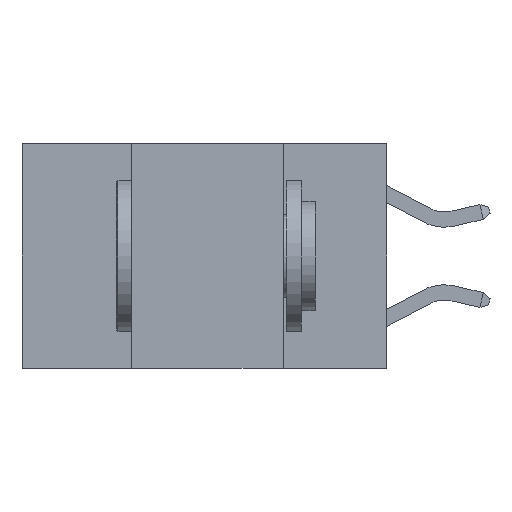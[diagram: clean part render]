
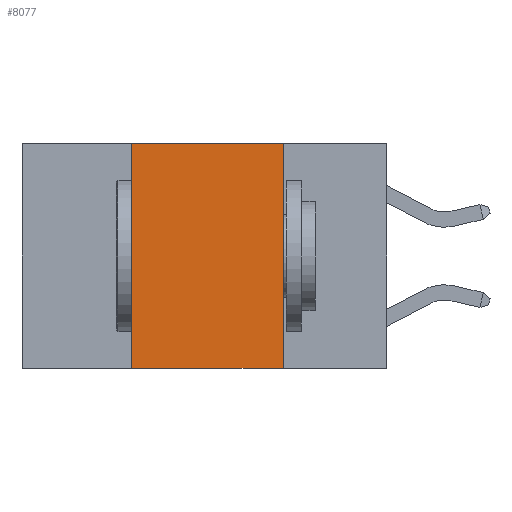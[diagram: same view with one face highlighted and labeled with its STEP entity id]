
A CAD part, left-side view. The second image highlights one B-rep face of the part: STEP entity #8077.
In plain terms, the highlighted planar face has unit normal (-1, 0, 0).
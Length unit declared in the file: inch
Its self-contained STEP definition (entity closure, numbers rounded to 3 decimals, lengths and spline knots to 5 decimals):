
#242 = CARTESIAN_POINT ( 'NONE',  ( 0., 0.17, 0. ) ) ;
#262 = CARTESIAN_POINT ( 'NONE',  ( 0., 0.6, 0. ) ) ;
#1111 = DIRECTION ( 'NONE',  ( 0., -1., 0. ) ) ;
#1276 = ORIENTED_EDGE ( 'NONE', *, *, #6042, .F. ) ;
#1295 = EDGE_LOOP ( 'NONE', ( #4457, #1276, #3113, #14697 ) ) ;
#1332 = CARTESIAN_POINT ( 'NONE',  ( 0., 0.6, 0. ) ) ;
#1393 = CARTESIAN_POINT ( 'NONE',  ( 0., 0.42, -0.37 ) ) ;
#2007 = DIRECTION ( 'NONE',  ( 0., 0., 1. ) ) ;
#3113 = ORIENTED_EDGE ( 'NONE', *, *, #12178, .F. ) ;
#3149 = CARTESIAN_POINT ( 'NONE',  ( 0., 0.42, 0. ) ) ;
#3438 = FACE_OUTER_BOUND ( 'NONE', #1295, .T. ) ;
#4027 = LINE ( 'NONE', #262, #12056 ) ;
#4457 = ORIENTED_EDGE ( 'NONE', *, *, #9704, .F. ) ;
#5697 = LINE ( 'NONE', #10254, #9868 ) ;
#6007 = DIRECTION ( 'NONE',  ( 1., 0., 0. ) ) ;
#6042 = EDGE_CURVE ( 'NONE', #13940, #7758, #4027, .T. ) ;
#6985 = LINE ( 'NONE', #3149, #11656 ) ;
#7730 = CARTESIAN_POINT ( 'NONE',  ( 0., 0.42, 0. ) ) ;
#7758 = VERTEX_POINT ( 'NONE', #242 ) ;
#8077 = ADVANCED_FACE ( 'NONE', ( #3438 ), #10652, .F. ) ;
#8408 = AXIS2_PLACEMENT_3D ( 'NONE', #1332, #6007, #13121 ) ;
#8499 = CARTESIAN_POINT ( 'NONE',  ( 0., 0.6, -0.37 ) ) ;
#9487 = EDGE_CURVE ( 'NONE', #11350, #12263, #10727, .T. ) ;
#9704 = EDGE_CURVE ( 'NONE', #7758, #12263, #5697, .T. ) ;
#9868 = VECTOR ( 'NONE', #13761, 39.37008 ) ;
#10254 = CARTESIAN_POINT ( 'NONE',  ( 0., 0.17, 0. ) ) ;
#10652 = PLANE ( 'NONE',  #8408 ) ;
#10727 = LINE ( 'NONE', #8499, #11844 ) ;
#11350 = VERTEX_POINT ( 'NONE', #1393 ) ;
#11656 = VECTOR ( 'NONE', #2007, 39.37008 ) ;
#11844 = VECTOR ( 'NONE', #1111, 39.37008 ) ;
#12056 = VECTOR ( 'NONE', #13537, 39.37008 ) ;
#12178 = EDGE_CURVE ( 'NONE', #11350, #13940, #6985, .T. ) ;
#12263 = VERTEX_POINT ( 'NONE', #13973 ) ;
#13121 = DIRECTION ( 'NONE',  ( 0., 0., -1. ) ) ;
#13537 = DIRECTION ( 'NONE',  ( 0., -1., 0. ) ) ;
#13761 = DIRECTION ( 'NONE',  ( 0., 0., -1. ) ) ;
#13940 = VERTEX_POINT ( 'NONE', #7730 ) ;
#13973 = CARTESIAN_POINT ( 'NONE',  ( 0., 0.17, -0.37 ) ) ;
#14697 = ORIENTED_EDGE ( 'NONE', *, *, #9487, .T. ) ;
